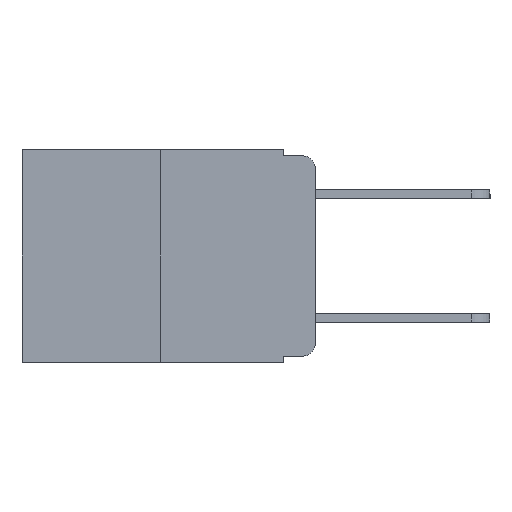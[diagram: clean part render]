
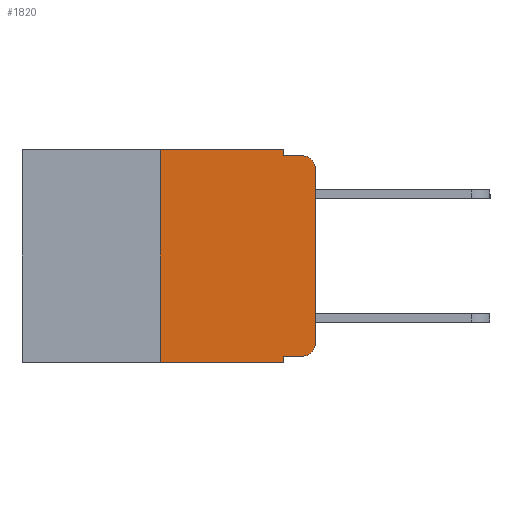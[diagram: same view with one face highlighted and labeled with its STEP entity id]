
A CAD part, left-side view. The second image highlights one B-rep face of the part: STEP entity #1820.
In plain terms, the highlighted planar face has unit normal (-1, 0, 0).
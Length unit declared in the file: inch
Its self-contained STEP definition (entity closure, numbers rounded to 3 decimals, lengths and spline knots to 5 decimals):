
#5 = DIRECTION ( 'NONE',  ( 0., 0., 1. ) ) ;
#185 = ORIENTED_EDGE ( 'NONE', *, *, #5131, .F. ) ;
#222 = CARTESIAN_POINT ( 'NONE',  ( 0., 0.02, -0.03 ) ) ;
#678 = PLANE ( 'NONE',  #18862 ) ;
#705 = CARTESIAN_POINT ( 'NONE',  ( 0., 0.473, -0.343 ) ) ;
#1820 = ADVANCED_FACE ( 'NONE', ( #8345 ), #678, .F. ) ;
#1962 = DIRECTION ( 'NONE',  ( 0., 0., -1. ) ) ;
#2471 = DIRECTION ( 'NONE',  ( 0., 0., -1. ) ) ;
#2542 = CARTESIAN_POINT ( 'NONE',  ( 0., 0., -0.03 ) ) ;
#2640 = VERTEX_POINT ( 'NONE', #19775 ) ;
#2820 = VECTOR ( 'NONE', #5, 39.37008 ) ;
#3128 = DIRECTION ( 'NONE',  ( 0., -1., 0. ) ) ;
#3243 = VECTOR ( 'NONE', #3128, 39.37008 ) ;
#3426 = EDGE_CURVE ( 'NONE', #8528, #11723, #3685, .T. ) ;
#3565 = DIRECTION ( 'NONE',  ( 0., 0., -1. ) ) ;
#3685 = LINE ( 'NONE', #11054, #16660 ) ;
#3860 = VECTOR ( 'NONE', #16750, 39.37008 ) ;
#4387 = CARTESIAN_POINT ( 'NONE',  ( 0., 0.051, -0.333 ) ) ;
#4644 = CARTESIAN_POINT ( 'NONE',  ( 0., 0.051, -0.343 ) ) ;
#4932 = DIRECTION ( 'NONE',  ( -1., 0., 0. ) ) ;
#5131 = EDGE_CURVE ( 'NONE', #16184, #11256, #18252, .T. ) ;
#5336 = DIRECTION ( 'NONE',  ( 0., -1., 0. ) ) ;
#5518 = CIRCLE ( 'NONE', #14209, 0.02 ) ;
#5832 = ORIENTED_EDGE ( 'NONE', *, *, #7185, .T. ) ;
#5875 = EDGE_LOOP ( 'NONE', ( #7146, #9957, #13021, #6910, #10821, #16928, #6125, #185, #13648, #5832 ) ) ;
#6125 = ORIENTED_EDGE ( 'NONE', *, *, #22003, .T. ) ;
#6586 = LINE ( 'NONE', #705, #10750 ) ;
#6656 = EDGE_CURVE ( 'NONE', #2640, #7913, #14053, .T. ) ;
#6898 = CARTESIAN_POINT ( 'NONE',  ( 0., 0.051, 0. ) ) ;
#6910 = ORIENTED_EDGE ( 'NONE', *, *, #17752, .F. ) ;
#7146 = ORIENTED_EDGE ( 'NONE', *, *, #3426, .T. ) ;
#7185 = EDGE_CURVE ( 'NONE', #10940, #8528, #16501, .T. ) ;
#7815 = EDGE_CURVE ( 'NONE', #9714, #9527, #22016, .T. ) ;
#7913 = VERTEX_POINT ( 'NONE', #6898 ) ;
#7938 = LINE ( 'NONE', #12907, #16811 ) ;
#8345 = FACE_OUTER_BOUND ( 'NONE', #5875, .T. ) ;
#8479 = CARTESIAN_POINT ( 'NONE',  ( 0., 0.051, -0.333 ) ) ;
#8528 = VERTEX_POINT ( 'NONE', #17326 ) ;
#8531 = LINE ( 'NONE', #4387, #3860 ) ;
#8566 = EDGE_CURVE ( 'NONE', #11723, #9527, #5518, .T. ) ;
#9483 = VERTEX_POINT ( 'NONE', #16757 ) ;
#9527 = VERTEX_POINT ( 'NONE', #9874 ) ;
#9714 = VERTEX_POINT ( 'NONE', #12518 ) ;
#9874 = CARTESIAN_POINT ( 'NONE',  ( 0., 0.02, -0.01 ) ) ;
#9892 = VECTOR ( 'NONE', #5336, 39.37008 ) ;
#9957 = ORIENTED_EDGE ( 'NONE', *, *, #8566, .T. ) ;
#10550 = DIRECTION ( 'NONE',  ( 0., 0., 1. ) ) ;
#10750 = VECTOR ( 'NONE', #12861, 39.37008 ) ;
#10821 = ORIENTED_EDGE ( 'NONE', *, *, #6656, .F. ) ;
#10843 = CARTESIAN_POINT ( 'NONE',  ( 0., 0.02, -0.333 ) ) ;
#10940 = VERTEX_POINT ( 'NONE', #10843 ) ;
#11054 = CARTESIAN_POINT ( 'NONE',  ( 0., 0., 0. ) ) ;
#11221 = AXIS2_PLACEMENT_3D ( 'NONE', #15529, #4932, #17303 ) ;
#11256 = VERTEX_POINT ( 'NONE', #4644 ) ;
#11723 = VERTEX_POINT ( 'NONE', #2542 ) ;
#12252 = CARTESIAN_POINT ( 'NONE',  ( 0., 0.25, 0. ) ) ;
#12472 = DIRECTION ( 'NONE',  ( -1., 0., 0. ) ) ;
#12518 = CARTESIAN_POINT ( 'NONE',  ( 0., 0.051, -0.01 ) ) ;
#12861 = DIRECTION ( 'NONE',  ( 0., -1., 0. ) ) ;
#12907 = CARTESIAN_POINT ( 'NONE',  ( 0., 0.051, 0. ) ) ;
#12995 = DIRECTION ( 'NONE',  ( 1., 0., 0. ) ) ;
#13021 = ORIENTED_EDGE ( 'NONE', *, *, #7815, .F. ) ;
#13648 = ORIENTED_EDGE ( 'NONE', *, *, #21451, .T. ) ;
#14053 = LINE ( 'NONE', #17723, #9892 ) ;
#14140 = CARTESIAN_POINT ( 'NONE',  ( 0., 0.051, 0. ) ) ;
#14209 = AXIS2_PLACEMENT_3D ( 'NONE', #222, #12472, #1962 ) ;
#14759 = DIRECTION ( 'NONE',  ( 0., 0., -1. ) ) ;
#15414 = CARTESIAN_POINT ( 'NONE',  ( 0., 0.051, -0.01 ) ) ;
#15439 = CARTESIAN_POINT ( 'NONE',  ( 0., 0.473, 0. ) ) ;
#15529 = CARTESIAN_POINT ( 'NONE',  ( 0., 0.02, -0.313 ) ) ;
#16184 = VERTEX_POINT ( 'NONE', #8479 ) ;
#16297 = VECTOR ( 'NONE', #3565, 39.37008 ) ;
#16304 = LINE ( 'NONE', #12252, #2820 ) ;
#16501 = CIRCLE ( 'NONE', #11221, 0.02 ) ;
#16660 = VECTOR ( 'NONE', #10550, 39.37008 ) ;
#16750 = DIRECTION ( 'NONE',  ( 0., -1., 0. ) ) ;
#16757 = CARTESIAN_POINT ( 'NONE',  ( 0., 0.25, -0.343 ) ) ;
#16811 = VECTOR ( 'NONE', #14759, 39.37008 ) ;
#16928 = ORIENTED_EDGE ( 'NONE', *, *, #21765, .F. ) ;
#17303 = DIRECTION ( 'NONE',  ( 0., 0., -1. ) ) ;
#17326 = CARTESIAN_POINT ( 'NONE',  ( 0., 0., -0.313 ) ) ;
#17723 = CARTESIAN_POINT ( 'NONE',  ( 0., 0.473, 0. ) ) ;
#17752 = EDGE_CURVE ( 'NONE', #7913, #9714, #7938, .T. ) ;
#18252 = LINE ( 'NONE', #14140, #16297 ) ;
#18862 = AXIS2_PLACEMENT_3D ( 'NONE', #15439, #12995, #2471 ) ;
#19775 = CARTESIAN_POINT ( 'NONE',  ( 0., 0.25, 0. ) ) ;
#21451 = EDGE_CURVE ( 'NONE', #16184, #10940, #8531, .T. ) ;
#21765 = EDGE_CURVE ( 'NONE', #9483, #2640, #16304, .T. ) ;
#22003 = EDGE_CURVE ( 'NONE', #9483, #11256, #6586, .T. ) ;
#22016 = LINE ( 'NONE', #15414, #3243 ) ;
